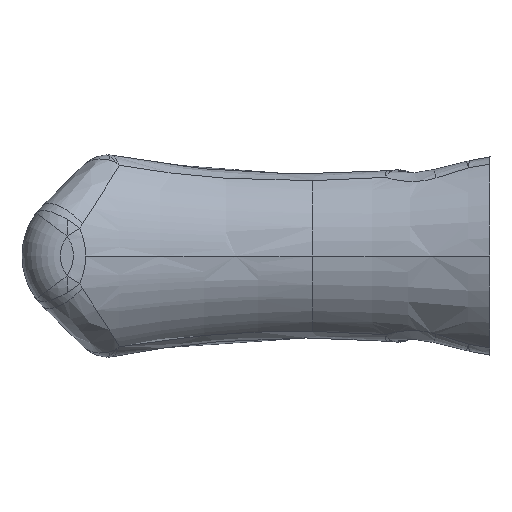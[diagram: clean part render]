
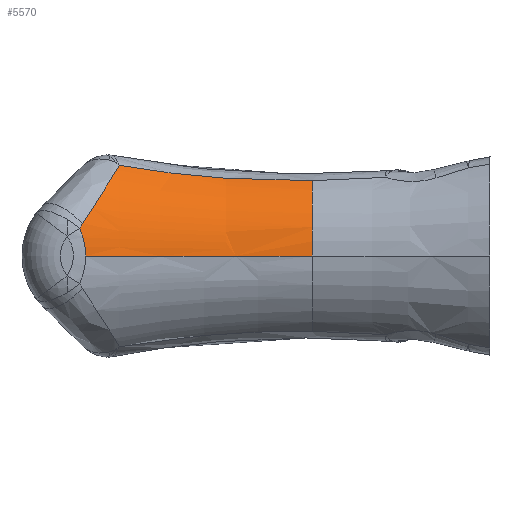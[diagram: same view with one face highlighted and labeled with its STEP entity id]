
A CAD part, left-side view. The second image highlights one B-rep face of the part: STEP entity #5570.
In plain terms, the highlighted toroidal (fillet/blend) face has major radius 208.719 mm and minor radius 185.111 mm.
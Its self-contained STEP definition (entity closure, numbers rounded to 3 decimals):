
#24 = CARTESIAN_POINT ( 'NONE',  ( -366.285, 17.37, 24.08 ) ) ;
#160 = VERTEX_POINT ( 'NONE', #4457 ) ;
#164 = CARTESIAN_POINT ( 'NONE',  ( -386.048, 72.657, 9.405 ) ) ;
#227 = CARTESIAN_POINT ( 'NONE',  ( -383.382, 70.421, 16.55 ) ) ;
#237 = CARTESIAN_POINT ( 'NONE',  ( -352.96, 13.135, 4.547 ) ) ;
#321 = AXIS2_PLACEMENT_3D ( 'NONE', #4922, #1461, #2009 ) ;
#516 = CARTESIAN_POINT ( 'NONE',  ( -366.608, 23.712, 24.165 ) ) ;
#544 = ORIENTED_EDGE ( 'NONE', *, *, #5825, .T. ) ;
#655 = CARTESIAN_POINT ( 'NONE',  ( -386.138, 72.092, 7.004 ) ) ;
#687 = CARTESIAN_POINT ( 'NONE',  ( -385.738, 73.267, 12.157 ) ) ;
#721 = CARTESIAN_POINT ( 'NONE',  ( -384.609, 71.798, 14.437 ) ) ;
#728 = DIRECTION ( 'NONE',  ( -1., 0., 0. ) ) ;
#850 = AXIS2_PLACEMENT_3D ( 'NONE', #2757, #6175, #3258 ) ;
#870 = VERTEX_POINT ( 'NONE', #4452 ) ;
#898 = TOROIDAL_SURFACE ( 'NONE', #321, 208.719, 185.111 ) ;
#975 = B_SPLINE_CURVE_WITH_KNOTS ( 'NONE', 3,
 ( #4611, #1194, #1696, #5101, #2193, #5602, #2668, #6090, #3172, #227, #3661, #721, #4152, #1214 ),
 .UNSPECIFIED., .F., .F.,
 ( 4, 2, 2, 2, 2, 2, 4 ),
 ( 0., 0.003, 0.006, 0.012, 0.017, 0.02, 0.023 ),
 .UNSPECIFIED. ) ;
#987 = CARTESIAN_POINT ( 'NONE',  ( -366.216, 15.251, 24.082 ) ) ;
#1012 = CARTESIAN_POINT ( 'NONE',  ( -367.104, 30.036, 24.392 ) ) ;
#1150 = CARTESIAN_POINT ( 'NONE',  ( -386.16, 71.952, 4.547 ) ) ;
#1194 = CARTESIAN_POINT ( 'NONE',  ( -373.106, 63.511, 27.589 ) ) ;
#1214 = CARTESIAN_POINT ( 'NONE',  ( -385.342, 72.744, 13.003 ) ) ;
#1461 = DIRECTION ( 'NONE',  ( 0., 1., 0. ) ) ;
#1510 = CARTESIAN_POINT ( 'NONE',  ( -367.765, 36.345, 24.763 ) ) ;
#1635 = VERTEX_POINT ( 'NONE', #3704 ) ;
#1642 = VERTEX_POINT ( 'NONE', #2736 ) ;
#1696 = CARTESIAN_POINT ( 'NONE',  ( -373.819, 63.827, 27.068 ) ) ;
#1714 = ORIENTED_EDGE ( 'NONE', *, *, #5059, .T. ) ;
#1733 = ORIENTED_EDGE ( 'NONE', *, *, #4283, .T. ) ;
#2009 = DIRECTION ( 'NONE',  ( -1., 0., 0. ) ) ;
#2011 = CARTESIAN_POINT ( 'NONE',  ( -369.183, 46.784, 25.683 ) ) ;
#2026 = EDGE_LOOP ( 'NONE', ( #3869, #544, #2840, #1714, #1733, #3304 ) ) ;
#2193 = CARTESIAN_POINT ( 'NONE',  ( -375.856, 64.831, 25.423 ) ) ;
#2493 = CARTESIAN_POINT ( 'NONE',  ( -371.452, 59.141, 27.362 ) ) ;
#2606 = CARTESIAN_POINT ( 'NONE',  ( -385.954, 73.255, 11.143 ) ) ;
#2668 = CARTESIAN_POINT ( 'NONE',  ( -378.922, 66.649, 22.479 ) ) ;
#2736 = CARTESIAN_POINT ( 'NONE',  ( -385.917, 73.495, 11.706 ) ) ;
#2757 = CARTESIAN_POINT ( 'NONE',  ( -561.679, 13.135, 4.547 ) ) ;
#2840 = ORIENTED_EDGE ( 'NONE', *, *, #4413, .T. ) ;
#2850 = EDGE_CURVE ( 'NONE', #1642, #5159, #5456, .T. ) ;
#2890 = VERTEX_POINT ( 'NONE', #5062 ) ;
#2895 = CIRCLE ( 'NONE', #5239, 23.608 ) ;
#3094 = CARTESIAN_POINT ( 'NONE',  ( -385.342, 72.744, 13.003 ) ) ;
#3107 = CARTESIAN_POINT ( 'NONE',  ( -385.988, 73.038, 10.571 ) ) ;
#3172 = CARTESIAN_POINT ( 'NONE',  ( -382.043, 69.091, 18.612 ) ) ;
#3258 = DIRECTION ( 'NONE',  ( -1., 0., 0. ) ) ;
#3304 = ORIENTED_EDGE ( 'NONE', *, *, #2850, .T. ) ;
#3462 = CARTESIAN_POINT ( 'NONE',  ( -366.481, 21.6, 24.121 ) ) ;
#3592 = CARTESIAN_POINT ( 'NONE',  ( -386.075, 72.491, 8.808 ) ) ;
#3661 = CARTESIAN_POINT ( 'NONE',  ( -383.807, 70.875, 15.849 ) ) ;
#3668 = DIRECTION ( 'NONE',  ( 0., 1., 0. ) ) ;
#3704 = CARTESIAN_POINT ( 'NONE',  ( -376.568, 13.135, 4.547 ) ) ;
#3834 = CARTESIAN_POINT ( 'NONE',  ( -366.179, 13.135, 24.108 ) ) ;
#3869 = ORIENTED_EDGE ( 'NONE', *, *, #5999, .T. ) ;
#3888 = CIRCLE ( 'NONE', #850, 185.111 ) ;
#3946 = CARTESIAN_POINT ( 'NONE',  ( -366.92, 27.93, 24.3 ) ) ;
#4082 = CARTESIAN_POINT ( 'NONE',  ( -386.16, 71.952, 5.785 ) ) ;
#4097 = CARTESIAN_POINT ( 'NONE',  ( -385.546, 73.018, 12.59 ) ) ;
#4119 = CARTESIAN_POINT ( 'NONE',  ( -385.917, 73.495, 11.706 ) ) ;
#4152 = CARTESIAN_POINT ( 'NONE',  ( -384.986, 72.267, 13.723 ) ) ;
#4202 = B_SPLINE_CURVE_WITH_KNOTS ( 'NONE', 3,
 ( #3094, #4097, #687, #4119 ),
 .UNSPECIFIED., .F., .F.,
 ( 4, 4 ),
 ( 0., 0.002 ),
 .UNSPECIFIED. ) ;
#4283 = EDGE_CURVE ( 'NONE', #160, #1642, #4202, .T. ) ;
#4413 = EDGE_CURVE ( 'NONE', #870, #2890, #5997, .T. ) ;
#4437 = CARTESIAN_POINT ( 'NONE',  ( -367.527, 34.243, 24.623 ) ) ;
#4452 = CARTESIAN_POINT ( 'NONE',  ( -366.179, 13.135, 24.108 ) ) ;
#4457 = CARTESIAN_POINT ( 'NONE',  ( -385.342, 72.744, 13.003 ) ) ;
#4611 = CARTESIAN_POINT ( 'NONE',  ( -372.371, 63.211, 28.086 ) ) ;
#4922 = CARTESIAN_POINT ( 'NONE',  ( -352.96, 13.135, 4.547 ) ) ;
#4923 = CARTESIAN_POINT ( 'NONE',  ( -368.555, 42.626, 25.256 ) ) ;
#5059 = EDGE_CURVE ( 'NONE', #2890, #160, #975, .T. ) ;
#5062 = CARTESIAN_POINT ( 'NONE',  ( -372.371, 63.211, 28.086 ) ) ;
#5101 = CARTESIAN_POINT ( 'NONE',  ( -375.196, 64.488, 25.983 ) ) ;
#5159 = VERTEX_POINT ( 'NONE', #5713 ) ;
#5239 = AXIS2_PLACEMENT_3D ( 'NONE', #237, #3668, #728 ) ;
#5418 = CARTESIAN_POINT ( 'NONE',  ( -370.631, 55.041, 26.736 ) ) ;
#5456 = B_SPLINE_CURVE_WITH_KNOTS ( 'NONE', 3,
 ( #6026, #2606, #3107, #164, #3592, #655, #4082, #1150 ),
 .UNSPECIFIED., .F., .F.,
 ( 4, 2, 2, 4 ),
 ( 0.011, 0.013, 0.015, 0.019 ),
 .UNSPECIFIED. ) ;
#5570 = ADVANCED_FACE ( 'NONE', ( #5957 ), #898, .F. ) ;
#5602 = CARTESIAN_POINT ( 'NONE',  ( -377.758, 65.894, 23.695 ) ) ;
#5713 = CARTESIAN_POINT ( 'NONE',  ( -386.16, 71.952, 4.547 ) ) ;
#5825 = EDGE_CURVE ( 'NONE', #1635, #870, #2895, .T. ) ;
#5905 = CARTESIAN_POINT ( 'NONE',  ( -372.371, 63.211, 28.086 ) ) ;
#5957 = FACE_OUTER_BOUND ( 'NONE', #2026, .T. ) ;
#5997 = B_SPLINE_CURVE_WITH_KNOTS ( 'NONE', 3,
 ( #3834, #987, #24, #3462, #516, #3946, #1012, #4437, #1510, #4923, #2011, #5418, #2493, #5905 ),
 .UNSPECIFIED., .F., .F.,
 ( 4, 2, 2, 2, 2, 2, 4 ),
 ( 0.048, 0.055, 0.061, 0.067, 0.074, 0.086, 0.099 ),
 .UNSPECIFIED. ) ;
#5999 = EDGE_CURVE ( 'NONE', #5159, #1635, #3888, .T. ) ;
#6026 = CARTESIAN_POINT ( 'NONE',  ( -385.917, 73.495, 11.706 ) ) ;
#6090 = CARTESIAN_POINT ( 'NONE',  ( -381.064, 68.248, 19.938 ) ) ;
#6175 = DIRECTION ( 'NONE',  ( 0., 0., -1. ) ) ;
